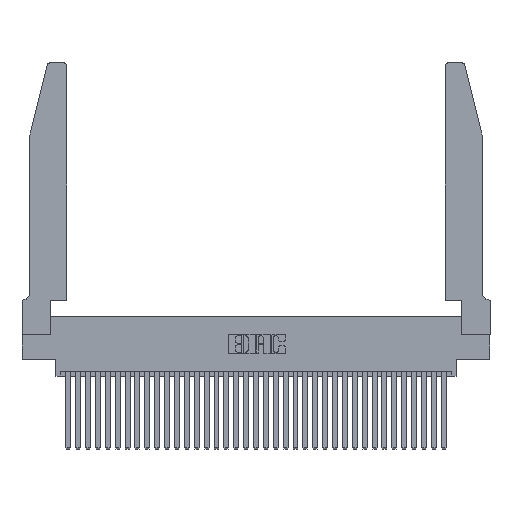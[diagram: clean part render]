
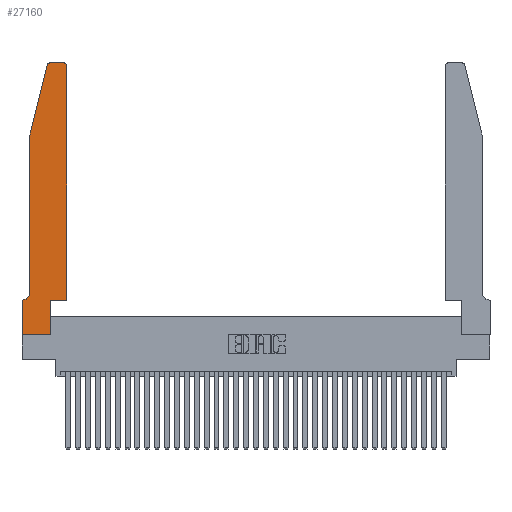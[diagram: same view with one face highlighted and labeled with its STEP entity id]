
A CAD part, top view. The second image highlights one B-rep face of the part: STEP entity #27160.
In plain terms, the highlighted planar face has unit normal (0, 0, 1).
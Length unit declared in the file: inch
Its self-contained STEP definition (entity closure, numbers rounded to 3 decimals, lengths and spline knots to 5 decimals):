
#331 = CIRCLE ( 'NONE', #23109, 0.03 ) ;
#731 = ORIENTED_EDGE ( 'NONE', *, *, #22181, .T. ) ;
#1065 = CARTESIAN_POINT ( 'NONE',  ( 0.4505, 0.35, 0.37 ) ) ;
#1608 = CARTESIAN_POINT ( 'NONE',  ( 0.284, 2.75, 0.37 ) ) ;
#2350 = CARTESIAN_POINT ( 'NONE',  ( 0.284, 2.72, 0.37 ) ) ;
#2380 = DIRECTION ( 'NONE',  ( 0., -1., 0. ) ) ;
#2572 = CARTESIAN_POINT ( 'NONE',  ( 0.2605, 2.75, 0.37 ) ) ;
#2973 = CIRCLE ( 'NONE', #15672, 0.03 ) ;
#3861 = CARTESIAN_POINT ( 'NONE',  ( 0.0755, 2., 0.37 ) ) ;
#4017 = DIRECTION ( 'NONE',  ( 1., 0., 0. ) ) ;
#4928 = EDGE_CURVE ( 'NONE', #5282, #6323, #15151, .T. ) ;
#4975 = VERTEX_POINT ( 'NONE', #32488 ) ;
#5282 = VERTEX_POINT ( 'NONE', #16458 ) ;
#5594 = LINE ( 'NONE', #12779, #19426 ) ;
#5671 = VECTOR ( 'NONE', #21426, 39.37008 ) ;
#5852 = EDGE_CURVE ( 'NONE', #32532, #16789, #19050, .T. ) ;
#6141 = ORIENTED_EDGE ( 'NONE', *, *, #11444, .T. ) ;
#6192 = DIRECTION ( 'NONE',  ( 0., 1., 0. ) ) ;
#6323 = VERTEX_POINT ( 'NONE', #21372 ) ;
#6880 = DIRECTION ( 'NONE',  ( 1., 0., 0. ) ) ;
#7115 = CARTESIAN_POINT ( 'NONE',  ( 0.2865, 0., 0.37 ) ) ;
#7648 = VECTOR ( 'NONE', #13028, 39.37008 ) ;
#7837 = CARTESIAN_POINT ( 'NONE',  ( 0.0755, 2., 0.37 ) ) ;
#8909 = EDGE_LOOP ( 'NONE', ( #11090, #13153, #6141, #21331, #18888, #20178, #18451, #15634, #21231, #14809, #12187, #731 ) ) ;
#8916 = CARTESIAN_POINT ( 'NONE',  ( 0.4505, 0.35, 0.37 ) ) ;
#8988 = DIRECTION ( 'NONE',  ( 1., 0., 0. ) ) ;
#9107 = CARTESIAN_POINT ( 'NONE',  ( 0., 0., 0.37 ) ) ;
#9126 = EDGE_CURVE ( 'NONE', #11748, #15308, #21836, .T. ) ;
#9938 = CARTESIAN_POINT ( 'NONE',  ( 0.0755, 0.42, 0.37 ) ) ;
#11090 = ORIENTED_EDGE ( 'NONE', *, *, #9126, .T. ) ;
#11444 = EDGE_CURVE ( 'NONE', #25794, #20543, #30518, .T. ) ;
#11539 = EDGE_CURVE ( 'NONE', #20543, #32532, #20014, .T. ) ;
#11748 = VERTEX_POINT ( 'NONE', #34991 ) ;
#11754 = DIRECTION ( 'NONE',  ( 0., 0., 1. ) ) ;
#12187 = ORIENTED_EDGE ( 'NONE', *, *, #18099, .T. ) ;
#12779 = CARTESIAN_POINT ( 'NONE',  ( 0.0755, 0.35, 0.37 ) ) ;
#13028 = DIRECTION ( 'NONE',  ( -0.239, -0.971, 0. ) ) ;
#13153 = ORIENTED_EDGE ( 'NONE', *, *, #34627, .T. ) ;
#13693 = VECTOR ( 'NONE', #8988, 39.37008 ) ;
#14075 = VECTOR ( 'NONE', #6880, 39.37008 ) ;
#14809 = ORIENTED_EDGE ( 'NONE', *, *, #18676, .T. ) ;
#14815 = DIRECTION ( 'NONE',  ( 0., 0., 1. ) ) ;
#14941 = DIRECTION ( 'NONE',  ( 1., 0., 0. ) ) ;
#15151 = LINE ( 'NONE', #35411, #27695 ) ;
#15308 = VERTEX_POINT ( 'NONE', #1608 ) ;
#15634 = ORIENTED_EDGE ( 'NONE', *, *, #24862, .T. ) ;
#15672 = AXIS2_PLACEMENT_3D ( 'NONE', #31296, #14815, #14941 ) ;
#16040 = VECTOR ( 'NONE', #22629, 39.37008 ) ;
#16458 = CARTESIAN_POINT ( 'NONE',  ( 0., 0.35, 0.37 ) ) ;
#16580 = DIRECTION ( 'NONE',  ( -1., 0., 0. ) ) ;
#16723 = CARTESIAN_POINT ( 'NONE',  ( 0.25487, 2.72718, 0.37 ) ) ;
#16789 = VERTEX_POINT ( 'NONE', #32818 ) ;
#16797 = VERTEX_POINT ( 'NONE', #8916 ) ;
#17175 = CARTESIAN_POINT ( 'NONE',  ( 0.0055, 0.42, 0.37 ) ) ;
#18099 = EDGE_CURVE ( 'NONE', #16797, #18902, #19207, .T. ) ;
#18451 = ORIENTED_EDGE ( 'NONE', *, *, #4928, .T. ) ;
#18676 = EDGE_CURVE ( 'NONE', #4975, #16797, #21416, .T. ) ;
#18888 = ORIENTED_EDGE ( 'NONE', *, *, #5852, .T. ) ;
#18893 = AXIS2_PLACEMENT_3D ( 'NONE', #17175, #25518, #20064 ) ;
#18902 = VERTEX_POINT ( 'NONE', #29438 ) ;
#18932 = VERTEX_POINT ( 'NONE', #7115 ) ;
#19050 = CIRCLE ( 'NONE', #18893, 0.07 ) ;
#19207 = LINE ( 'NONE', #1065, #29939 ) ;
#19426 = VECTOR ( 'NONE', #31903, 39.37008 ) ;
#20014 = LINE ( 'NONE', #21304, #5671 ) ;
#20064 = DIRECTION ( 'NONE',  ( -1., 0., 0. ) ) ;
#20078 = CARTESIAN_POINT ( 'NONE',  ( 0.2865, 0.35, 0.37 ) ) ;
#20178 = ORIENTED_EDGE ( 'NONE', *, *, #22823, .T. ) ;
#20543 = VERTEX_POINT ( 'NONE', #3861 ) ;
#20656 = CARTESIAN_POINT ( 'NONE',  ( 0.4505, 0.35, 0.37 ) ) ;
#21231 = ORIENTED_EDGE ( 'NONE', *, *, #21413, .T. ) ;
#21304 = CARTESIAN_POINT ( 'NONE',  ( 0.0755, 2., 0.37 ) ) ;
#21331 = ORIENTED_EDGE ( 'NONE', *, *, #11539, .T. ) ;
#21372 = CARTESIAN_POINT ( 'NONE',  ( 0., 0., 0.37 ) ) ;
#21413 = EDGE_CURVE ( 'NONE', #18932, #4975, #33656, .T. ) ;
#21416 = LINE ( 'NONE', #20656, #14075 ) ;
#21426 = DIRECTION ( 'NONE',  ( 0., -1., 0. ) ) ;
#21836 = LINE ( 'NONE', #2572, #27035 ) ;
#21870 = LINE ( 'NONE', #9107, #13693 ) ;
#22181 = EDGE_CURVE ( 'NONE', #18902, #11748, #2973, .T. ) ;
#22629 = DIRECTION ( 'NONE',  ( 0., 1., 0. ) ) ;
#22823 = EDGE_CURVE ( 'NONE', #16789, #5282, #5594, .T. ) ;
#23109 = AXIS2_PLACEMENT_3D ( 'NONE', #2350, #26980, #32865 ) ;
#24862 = EDGE_CURVE ( 'NONE', #6323, #18932, #21870, .T. ) ;
#25518 = DIRECTION ( 'NONE',  ( 0., 0., -1. ) ) ;
#25794 = VERTEX_POINT ( 'NONE', #16723 ) ;
#25881 = CARTESIAN_POINT ( 'NONE',  ( 0., 0.35, 0.37 ) ) ;
#26980 = DIRECTION ( 'NONE',  ( 0., 0., 1. ) ) ;
#27035 = VECTOR ( 'NONE', #16580, 39.37008 ) ;
#27160 = ADVANCED_FACE ( 'NONE', ( #35418 ), #31117, .T. ) ;
#27545 = AXIS2_PLACEMENT_3D ( 'NONE', #25881, #11754, #4017 ) ;
#27695 = VECTOR ( 'NONE', #2380, 39.37008 ) ;
#29438 = CARTESIAN_POINT ( 'NONE',  ( 0.4505, 2.72, 0.37 ) ) ;
#29939 = VECTOR ( 'NONE', #6192, 39.37008 ) ;
#30518 = LINE ( 'NONE', #7837, #7648 ) ;
#31117 = PLANE ( 'NONE',  #27545 ) ;
#31296 = CARTESIAN_POINT ( 'NONE',  ( 0.4205, 2.72, 0.37 ) ) ;
#31903 = DIRECTION ( 'NONE',  ( -1., 0., 0. ) ) ;
#32488 = CARTESIAN_POINT ( 'NONE',  ( 0.2865, 0.35, 0.37 ) ) ;
#32532 = VERTEX_POINT ( 'NONE', #9938 ) ;
#32818 = CARTESIAN_POINT ( 'NONE',  ( 0.0055, 0.35, 0.37 ) ) ;
#32865 = DIRECTION ( 'NONE',  ( 1., 0., 0. ) ) ;
#33656 = LINE ( 'NONE', #20078, #16040 ) ;
#34627 = EDGE_CURVE ( 'NONE', #15308, #25794, #331, .T. ) ;
#34991 = CARTESIAN_POINT ( 'NONE',  ( 0.4205, 2.75, 0.37 ) ) ;
#35411 = CARTESIAN_POINT ( 'NONE',  ( 0., 0., 0.37 ) ) ;
#35418 = FACE_OUTER_BOUND ( 'NONE', #8909, .T. ) ;
